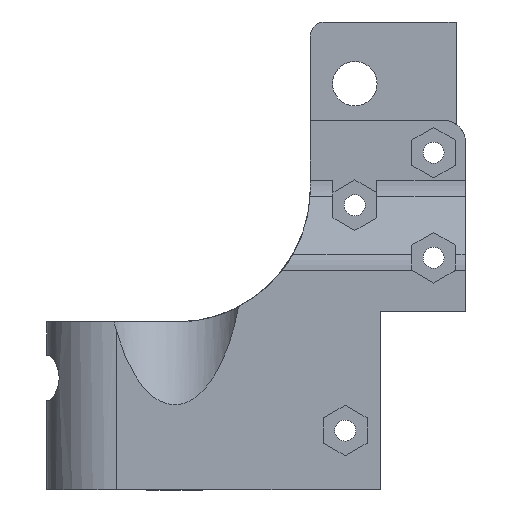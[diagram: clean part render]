
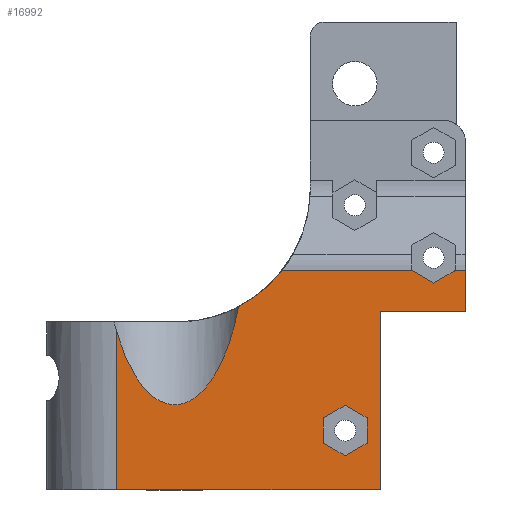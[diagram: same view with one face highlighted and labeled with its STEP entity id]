
A CAD part, left-side view. The second image highlights one B-rep face of the part: STEP entity #16992.
In plain terms, the highlighted planar face has unit normal (-1, 0, 0).
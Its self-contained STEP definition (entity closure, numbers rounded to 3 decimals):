
#99 = VECTOR ( 'NONE', #29270, 1000. ) ;
#228 = LINE ( 'NONE', #19582, #99 ) ;
#402 = ORIENTED_EDGE ( 'NONE', *, *, #22505, .F. ) ;
#662 = DIRECTION ( 'NONE',  ( 0., 1., 0. ) ) ;
#1086 = DIRECTION ( 'NONE',  ( 0., 0., -1. ) ) ;
#1529 = CARTESIAN_POINT ( 'NONE',  ( -25., 14.266, 5.203 ) ) ;
#1707 = CARTESIAN_POINT ( 'NONE',  ( -25., 19.225, 22.598 ) ) ;
#2242 = ORIENTED_EDGE ( 'NONE', *, *, #7206, .F. ) ;
#2280 = VERTEX_POINT ( 'NONE', #2333 ) ;
#2333 = CARTESIAN_POINT ( 'NONE',  ( -25., -13.405, 4.882 ) ) ;
#2371 = ORIENTED_EDGE ( 'NONE', *, *, #25843, .T. ) ;
#2431 = LINE ( 'NONE', #12265, #15310 ) ;
#2588 = VECTOR ( 'NONE', #14228, 1000. ) ;
#2967 = EDGE_CURVE ( 'NONE', #27438, #13581, #5689, .T. ) ;
#3588 = VERTEX_POINT ( 'NONE', #19171 ) ;
#3964 = CARTESIAN_POINT ( 'NONE',  ( -25., -44.561, 25.53 ) ) ;
#4183 = CARTESIAN_POINT ( 'NONE',  ( -25., -30.561, 32.5 ) ) ;
#4256 = CARTESIAN_POINT ( 'NONE',  ( -25., -13.405, 12.098 ) ) ;
#4416 = ORIENTED_EDGE ( 'NONE', *, *, #27608, .F. ) ;
#4510 = CARTESIAN_POINT ( 'NONE',  ( -25., -29.225, 0. ) ) ;
#4696 = CARTESIAN_POINT ( 'NONE',  ( -25., -13.405, 4.882 ) ) ;
#4744 = EDGE_CURVE ( 'NONE', #27174, #23465, #2431, .T. ) ;
#4924 = ORIENTED_EDGE ( 'NONE', *, *, #27531, .F. ) ;
#4951 = VERTEX_POINT ( 'NONE', #26614 ) ;
#5006 = DIRECTION ( 'NONE',  ( 0., 0., 1. ) ) ;
#5265 = ORIENTED_EDGE ( 'NONE', *, *, #20934, .T. ) ;
#5497 = CARTESIAN_POINT ( 'NONE',  ( -25., -30.561, 31.322 ) ) ;
#5511 = EDGE_CURVE ( 'NONE', #15098, #4951, #31049, .T. ) ;
#5689 = LINE ( 'NONE', #7911, #8295 ) ;
#5811 = ORIENTED_EDGE ( 'NONE', *, *, #15835, .F. ) ;
#6019 = CARTESIAN_POINT ( 'NONE',  ( -25., -16.53, 10.294 ) ) ;
#6097 = FACE_OUTER_BOUND ( 'NONE', #11040, .T. ) ;
#6277 = ORIENTED_EDGE ( 'NONE', *, *, #22215, .T. ) ;
#6297 = CARTESIAN_POINT ( 'NONE',  ( -25., 19.225, 107.64 ) ) ;
#6487 = CARTESIAN_POINT ( 'NONE',  ( -25., -13.405, 12.098 ) ) ;
#6750 = DIRECTION ( 'NONE',  ( 1., 0., 0. ) ) ;
#6980 = EDGE_LOOP ( 'NONE', ( #14706, #14028, #402, #27722, #12718, #4416 ) ) ;
#7157 = CARTESIAN_POINT ( 'NONE',  ( -25., -62.24, 50.456 ) ) ;
#7197 = VECTOR ( 'NONE', #25228, 1000. ) ;
#7206 = EDGE_CURVE ( 'NONE', #27174, #10656, #9247, .T. ) ;
#7264 = ORIENTED_EDGE ( 'NONE', *, *, #24338, .F. ) ;
#7911 = CARTESIAN_POINT ( 'NONE',  ( -25., -18.405, 0. ) ) ;
#8247 = EDGE_CURVE ( 'NONE', #25983, #16624, #16141, .T. ) ;
#8295 = VECTOR ( 'NONE', #1086, 1000. ) ;
#8497 = VERTEX_POINT ( 'NONE', #4256 ) ;
#8636 = CARTESIAN_POINT ( 'NONE',  ( -25., -29.225, 107.64 ) ) ;
#8819 = ORIENTED_EDGE ( 'NONE', *, *, #2967, .F. ) ;
#9165 = ORIENTED_EDGE ( 'NONE', *, *, #10797, .F. ) ;
#9247 = LINE ( 'NONE', #4183, #11811 ) ;
#9378 = CARTESIAN_POINT ( 'NONE',  ( -25., -5.237, 31.322 ) ) ;
#9405 = EDGE_CURVE ( 'NONE', #10400, #24092, #31205, .T. ) ;
#9590 = CARTESIAN_POINT ( 'NONE',  ( -25., -18.405, 25.53 ) ) ;
#9923 = DIRECTION ( 'NONE',  ( 0., 0.866, 0.5 ) ) ;
#10400 = VERTEX_POINT ( 'NONE', #18603 ) ;
#10455 = CARTESIAN_POINT ( 'NONE',  ( -25., -10.28, 10.294 ) ) ;
#10656 = VERTEX_POINT ( 'NONE', #18445 ) ;
#10746 = VECTOR ( 'NONE', #26366, 1000. ) ;
#10797 = EDGE_CURVE ( 'NONE', #3588, #23465, #28763, .T. ) ;
#10872 = CARTESIAN_POINT ( 'NONE',  ( -25., -10.28, 6.686 ) ) ;
#11040 = EDGE_LOOP ( 'NONE', ( #2242, #28548, #9165, #4924, #2371, #18038, #5811, #6277, #5265, #8819, #7264 ) ) ;
#11386 = CARTESIAN_POINT ( 'NONE',  ( -25., 1.808, 26.163 ) ) ;
#11712 = VECTOR ( 'NONE', #26897, 1000. ) ;
#11811 = VECTOR ( 'NONE', #13534, 1000. ) ;
#12265 = CARTESIAN_POINT ( 'NONE',  ( -25., -29.146, 31.322 ) ) ;
#12266 = VECTOR ( 'NONE', #24350, 1000. ) ;
#12629 = EDGE_CURVE ( 'NONE', #2280, #10400, #26445, .T. ) ;
#12718 = ORIENTED_EDGE ( 'NONE', *, *, #12629, .F. ) ;
#13534 = DIRECTION ( 'NONE',  ( 0., 0., -1. ) ) ;
#13563 = FACE_BOUND ( 'NONE', #6980, .T. ) ;
#13581 = VERTEX_POINT ( 'NONE', #24980 ) ;
#13640 = DIRECTION ( 'NONE',  ( 0., 1., 0. ) ) ;
#14028 = ORIENTED_EDGE ( 'NONE', *, *, #26462, .F. ) ;
#14228 = DIRECTION ( 'NONE',  ( 0., 0., -1. ) ) ;
#14668 = CARTESIAN_POINT ( 'NONE',  ( -25., 5.392, 47.682 ) ) ;
#14706 = ORIENTED_EDGE ( 'NONE', *, *, #8247, .F. ) ;
#15039 = DIRECTION ( 'NONE',  ( 0., 0., 1. ) ) ;
#15098 = VERTEX_POINT ( 'NONE', #25084 ) ;
#15310 = VECTOR ( 'NONE', #662, 1000. ) ;
#15552 = LINE ( 'NONE', #3964, #26949 ) ;
#15835 = EDGE_CURVE ( 'NONE', #28601, #15098, #18435, .T. ) ;
#16102 = DIRECTION ( 'NONE',  ( 0., 0., -1. ) ) ;
#16132 = LINE ( 'NONE', #6297, #2588 ) ;
#16141 = LINE ( 'NONE', #30421, #29556 ) ;
#16292 = LINE ( 'NONE', #21836, #25920 ) ;
#16624 = VERTEX_POINT ( 'NONE', #10872 ) ;
#16844 = CARTESIAN_POINT ( 'NONE',  ( -25., -29.098, 31.322 ) ) ;
#16992 = ADVANCED_FACE ( 'NONE', ( #13563, #6097 ), #23247, .F. ) ;
#17049 = LINE ( 'NONE', #14668, #12266 ) ;
#18038 = ORIENTED_EDGE ( 'NONE', *, *, #5511, .F. ) ;
#18435 =( BOUNDED_CURVE ( )  B_SPLINE_CURVE ( 3, ( #1707, #1529, #28688, #11386 ),
 .UNSPECIFIED., .F., .T. ) 
 B_SPLINE_CURVE_WITH_KNOTS ( ( 4, 4 ),
 ( 5.306, 7.433 ),
 .UNSPECIFIED. ) 
 CURVE ( )  GEOMETRIC_REPRESENTATION_ITEM ( )  RATIONAL_B_SPLINE_CURVE ( ( 1., 0.657, 0.657, 1. ) ) 
 REPRESENTATION_ITEM ( '' )  );
#18445 = CARTESIAN_POINT ( 'NONE',  ( -25., -30.561, 25.53 ) ) ;
#18603 = CARTESIAN_POINT ( 'NONE',  ( -25., -16.53, 6.686 ) ) ;
#19171 = CARTESIAN_POINT ( 'NONE',  ( -25., -26.021, 29.546 ) ) ;
#19370 = AXIS2_PLACEMENT_3D ( 'NONE', #27597, #22188, #15039 ) ;
#19582 = CARTESIAN_POINT ( 'NONE',  ( -25., -10.28, 6.686 ) ) ;
#20934 = EDGE_CURVE ( 'NONE', #25811, #13581, #30860, .T. ) ;
#21209 = CARTESIAN_POINT ( 'NONE',  ( -25., -16.53, 6.686 ) ) ;
#21438 = CARTESIAN_POINT ( 'NONE',  ( -25., 19.225, 0. ) ) ;
#21455 = DIRECTION ( 'NONE',  ( 0., -0.866, 0.5 ) ) ;
#21836 = CARTESIAN_POINT ( 'NONE',  ( -25., -16.53, 10.294 ) ) ;
#22188 = DIRECTION ( 'NONE',  ( -1., 0., 0. ) ) ;
#22215 = EDGE_CURVE ( 'NONE', #28601, #25811, #16132, .T. ) ;
#22489 = VECTOR ( 'NONE', #21455, 1000. ) ;
#22505 = EDGE_CURVE ( 'NONE', #24092, #8497, #16292, .T. ) ;
#23230 = VERTEX_POINT ( 'NONE', #24000 ) ;
#23247 = PLANE ( 'NONE',  #25442 ) ;
#23465 = VERTEX_POINT ( 'NONE', #16844 ) ;
#24000 = CARTESIAN_POINT ( 'NONE',  ( -25., -22.945, 31.322 ) ) ;
#24092 = VERTEX_POINT ( 'NONE', #6019 ) ;
#24338 = EDGE_CURVE ( 'NONE', #10656, #27438, #15552, .T. ) ;
#24350 = DIRECTION ( 'NONE',  ( 0., -0.866, -0.5 ) ) ;
#24980 = CARTESIAN_POINT ( 'NONE',  ( -25., -18.405, 0. ) ) ;
#25084 = CARTESIAN_POINT ( 'NONE',  ( -25., 1.808, 26.163 ) ) ;
#25228 = DIRECTION ( 'NONE',  ( 0., 0.866, -0.5 ) ) ;
#25442 = AXIS2_PLACEMENT_3D ( 'NONE', #8636, #6750, #16102 ) ;
#25811 = VERTEX_POINT ( 'NONE', #21438 ) ;
#25833 = DIRECTION ( 'NONE',  ( 0., 0., -1. ) ) ;
#25843 = EDGE_CURVE ( 'NONE', #23230, #4951, #31129, .T. ) ;
#25853 = LINE ( 'NONE', #6487, #7197 ) ;
#25920 = VECTOR ( 'NONE', #9923, 1000. ) ;
#25970 = VECTOR ( 'NONE', #28482, 1000. ) ;
#25983 = VERTEX_POINT ( 'NONE', #10455 ) ;
#26017 = VECTOR ( 'NONE', #5006, 1000. ) ;
#26366 = DIRECTION ( 'NONE',  ( 0., 1., 0. ) ) ;
#26445 = LINE ( 'NONE', #4696, #11712 ) ;
#26462 = EDGE_CURVE ( 'NONE', #8497, #25983, #25853, .T. ) ;
#26614 = CARTESIAN_POINT ( 'NONE',  ( -25., -4.387, 31.322 ) ) ;
#26897 = DIRECTION ( 'NONE',  ( 0., -0.866, 0.5 ) ) ;
#26949 = VECTOR ( 'NONE', #13640, 1000. ) ;
#27174 = VERTEX_POINT ( 'NONE', #5497 ) ;
#27438 = VERTEX_POINT ( 'NONE', #9590 ) ;
#27531 = EDGE_CURVE ( 'NONE', #23230, #3588, #17049, .T. ) ;
#27597 = CARTESIAN_POINT ( 'NONE',  ( -25., 10.625, 43.05 ) ) ;
#27608 = EDGE_CURVE ( 'NONE', #16624, #2280, #228, .T. ) ;
#27722 = ORIENTED_EDGE ( 'NONE', *, *, #9405, .F. ) ;
#28482 = DIRECTION ( 'NONE',  ( 0., -1., 0. ) ) ;
#28548 = ORIENTED_EDGE ( 'NONE', *, *, #4744, .T. ) ;
#28601 = VERTEX_POINT ( 'NONE', #29960 ) ;
#28688 = CARTESIAN_POINT ( 'NONE',  ( -25., 5.431, 7.012 ) ) ;
#28763 = LINE ( 'NONE', #7157, #22489 ) ;
#29270 = DIRECTION ( 'NONE',  ( 0., -0.866, -0.5 ) ) ;
#29556 = VECTOR ( 'NONE', #25833, 1000. ) ;
#29960 = CARTESIAN_POINT ( 'NONE',  ( -25., 19.225, 22.598 ) ) ;
#30421 = CARTESIAN_POINT ( 'NONE',  ( -25., -10.28, 10.294 ) ) ;
#30860 = LINE ( 'NONE', #4510, #25970 ) ;
#31049 = CIRCLE ( 'NONE', #19370, 19.05 ) ;
#31129 = LINE ( 'NONE', #9378, #10746 ) ;
#31205 = LINE ( 'NONE', #21209, #26017 ) ;
